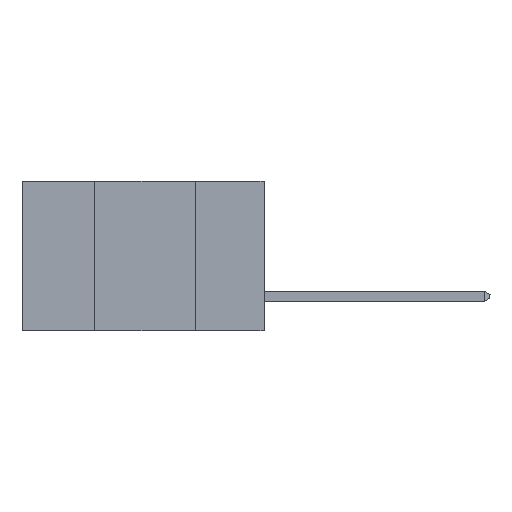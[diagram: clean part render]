
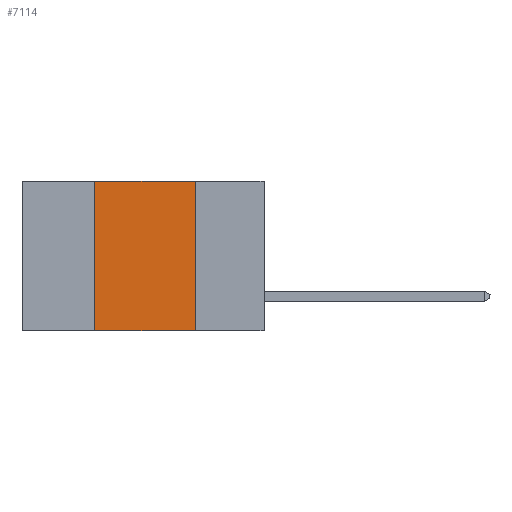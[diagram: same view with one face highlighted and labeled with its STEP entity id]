
A CAD part, left-side view. The second image highlights one B-rep face of the part: STEP entity #7114.
In plain terms, the highlighted planar face has unit normal (-1, 0, 0).
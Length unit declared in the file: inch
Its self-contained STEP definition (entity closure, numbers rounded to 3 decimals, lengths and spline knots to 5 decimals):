
#1127 = FACE_OUTER_BOUND ( 'NONE', #2130, .T. ) ;
#1502 = CARTESIAN_POINT ( 'NONE',  ( 0., 0.42, 0. ) ) ;
#1754 = ORIENTED_EDGE ( 'NONE', *, *, #12459, .F. ) ;
#1994 = ORIENTED_EDGE ( 'NONE', *, *, #10229, .T. ) ;
#2130 = EDGE_LOOP ( 'NONE', ( #11387, #15347, #1754, #1994 ) ) ;
#2882 = DIRECTION ( 'NONE',  ( 0., -1., 0. ) ) ;
#3120 = EDGE_CURVE ( 'NONE', #9951, #4287, #9568, .T. ) ;
#4089 = CARTESIAN_POINT ( 'NONE',  ( 0., 0.6, 0. ) ) ;
#4287 = VERTEX_POINT ( 'NONE', #14637 ) ;
#4343 = LINE ( 'NONE', #7001, #16524 ) ;
#4565 = CARTESIAN_POINT ( 'NONE',  ( 0., 0.17, -0.37 ) ) ;
#4762 = CARTESIAN_POINT ( 'NONE',  ( 0., 0.6, 0. ) ) ;
#4843 = PLANE ( 'NONE',  #7526 ) ;
#5583 = EDGE_CURVE ( 'NONE', #11860, #9951, #14325, .T. ) ;
#7001 = CARTESIAN_POINT ( 'NONE',  ( 0., 0.42, -0.37 ) ) ;
#7069 = VECTOR ( 'NONE', #11103, 39.37008 ) ;
#7111 = CARTESIAN_POINT ( 'NONE',  ( 0., 0.6, -0.37 ) ) ;
#7114 = ADVANCED_FACE ( 'NONE', ( #1127 ), #4843, .F. ) ;
#7526 = AXIS2_PLACEMENT_3D ( 'NONE', #4762, #11474, #8909 ) ;
#8199 = VECTOR ( 'NONE', #2882, 39.37008 ) ;
#8909 = DIRECTION ( 'NONE',  ( 0., 0., -1. ) ) ;
#9568 = LINE ( 'NONE', #4565, #7069 ) ;
#9951 = VERTEX_POINT ( 'NONE', #12347 ) ;
#10229 = EDGE_CURVE ( 'NONE', #12304, #4287, #10755, .T. ) ;
#10755 = LINE ( 'NONE', #7111, #8199 ) ;
#11103 = DIRECTION ( 'NONE',  ( 0., 0., -1. ) ) ;
#11387 = ORIENTED_EDGE ( 'NONE', *, *, #3120, .F. ) ;
#11474 = DIRECTION ( 'NONE',  ( 1., 0., 0. ) ) ;
#11860 = VERTEX_POINT ( 'NONE', #1502 ) ;
#12304 = VERTEX_POINT ( 'NONE', #16515 ) ;
#12347 = CARTESIAN_POINT ( 'NONE',  ( 0., 0.17, 0. ) ) ;
#12459 = EDGE_CURVE ( 'NONE', #12304, #11860, #4343, .T. ) ;
#13071 = DIRECTION ( 'NONE',  ( 0., -1., 0. ) ) ;
#14325 = LINE ( 'NONE', #4089, #15032 ) ;
#14637 = CARTESIAN_POINT ( 'NONE',  ( 0., 0.17, -0.37 ) ) ;
#14661 = DIRECTION ( 'NONE',  ( 0., 0., 1. ) ) ;
#15032 = VECTOR ( 'NONE', #13071, 39.37008 ) ;
#15347 = ORIENTED_EDGE ( 'NONE', *, *, #5583, .F. ) ;
#16515 = CARTESIAN_POINT ( 'NONE',  ( 0., 0.42, -0.37 ) ) ;
#16524 = VECTOR ( 'NONE', #14661, 39.37008 ) ;
